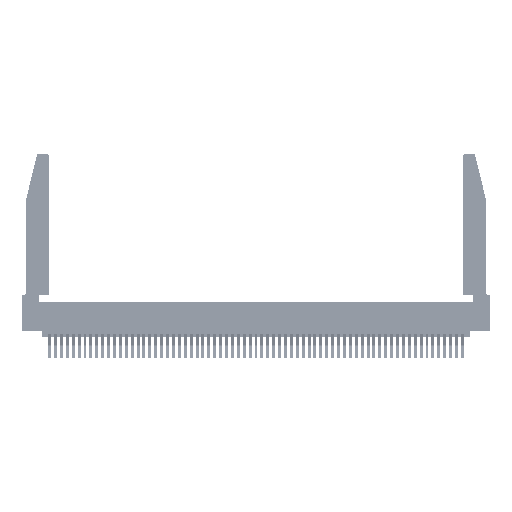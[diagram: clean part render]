
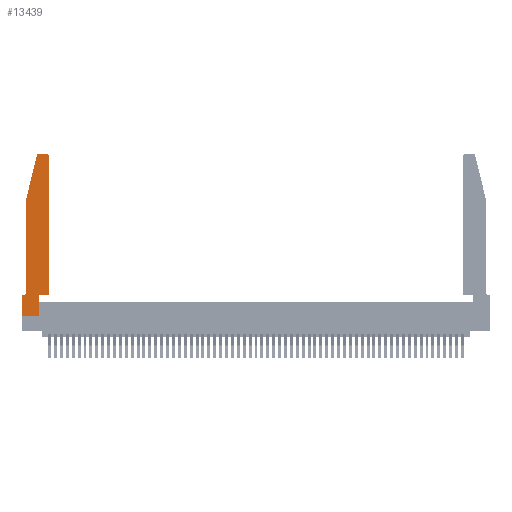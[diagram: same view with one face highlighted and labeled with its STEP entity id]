
A CAD part, top view. The second image highlights one B-rep face of the part: STEP entity #13439.
In plain terms, the highlighted planar face has unit normal (0, 0, 1).
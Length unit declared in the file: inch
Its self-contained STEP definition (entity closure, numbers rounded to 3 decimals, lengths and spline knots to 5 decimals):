
#87 = ORIENTED_EDGE ( 'NONE', *, *, #21274, .T. ) ;
#419 = VECTOR ( 'NONE', #16377, 39.37008 ) ;
#1144 = VERTEX_POINT ( 'NONE', #14905 ) ;
#1834 = CARTESIAN_POINT ( 'NONE',  ( 0.0055, 0.35, 0.37 ) ) ;
#1866 = LINE ( 'NONE', #2980, #419 ) ;
#2343 = EDGE_CURVE ( 'NONE', #43967, #1144, #30442, .T. ) ;
#2518 = CARTESIAN_POINT ( 'NONE',  ( 0.2865, 0.35, 0.37 ) ) ;
#2842 = ORIENTED_EDGE ( 'NONE', *, *, #17449, .T. ) ;
#2980 = CARTESIAN_POINT ( 'NONE',  ( 0.4505, 0.35, 0.37 ) ) ;
#3191 = LINE ( 'NONE', #33916, #36952 ) ;
#3892 = CARTESIAN_POINT ( 'NONE',  ( 0., 0.35, 0.37 ) ) ;
#4435 = DIRECTION ( 'NONE',  ( 1., 0., 0. ) ) ;
#4723 = CARTESIAN_POINT ( 'NONE',  ( 0.0755, 0.35, 0.37 ) ) ;
#4986 = EDGE_CURVE ( 'NONE', #23277, #34594, #48489, .T. ) ;
#5248 = CIRCLE ( 'NONE', #18675, 0.03 ) ;
#5651 = CARTESIAN_POINT ( 'NONE',  ( 0., 0., 0.37 ) ) ;
#5945 = CARTESIAN_POINT ( 'NONE',  ( 0.4205, 2.75, 0.37 ) ) ;
#7205 = ORIENTED_EDGE ( 'NONE', *, *, #27578, .T. ) ;
#7574 = DIRECTION ( 'NONE',  ( 0., -1., 0. ) ) ;
#7588 = PLANE ( 'NONE',  #23251 ) ;
#9173 = DIRECTION ( 'NONE',  ( -1., 0., 0. ) ) ;
#9368 = CARTESIAN_POINT ( 'NONE',  ( 0.284, 2.72, 0.37 ) ) ;
#11426 = CARTESIAN_POINT ( 'NONE',  ( 0.4505, 2.72, 0.37 ) ) ;
#11681 = ORIENTED_EDGE ( 'NONE', *, *, #2343, .T. ) ;
#11766 = ORIENTED_EDGE ( 'NONE', *, *, #26787, .T. ) ;
#12074 = CARTESIAN_POINT ( 'NONE',  ( 0., 0.35, 0.37 ) ) ;
#12823 = CIRCLE ( 'NONE', #55112, 0.03 ) ;
#13439 = ADVANCED_FACE ( 'NONE', ( #52415 ), #7588, .T. ) ;
#13842 = DIRECTION ( 'NONE',  ( 1., 0., 0. ) ) ;
#14390 = DIRECTION ( 'NONE',  ( -0.239, -0.971, 0. ) ) ;
#14905 = CARTESIAN_POINT ( 'NONE',  ( 0.0755, 2., 0.37 ) ) ;
#14991 = VECTOR ( 'NONE', #24948, 39.37008 ) ;
#16377 = DIRECTION ( 'NONE',  ( 0., 1., 0. ) ) ;
#16488 = CARTESIAN_POINT ( 'NONE',  ( 0.0755, 0.42, 0.37 ) ) ;
#16492 = DIRECTION ( 'NONE',  ( 1., 0., 0. ) ) ;
#17449 = EDGE_CURVE ( 'NONE', #37612, #43967, #12823, .T. ) ;
#18675 = AXIS2_PLACEMENT_3D ( 'NONE', #40758, #30841, #4435 ) ;
#18746 = VECTOR ( 'NONE', #14390, 39.37008 ) ;
#18855 = VERTEX_POINT ( 'NONE', #45283 ) ;
#19346 = VECTOR ( 'NONE', #50875, 39.37008 ) ;
#19733 = CARTESIAN_POINT ( 'NONE',  ( 0.284, 2.75, 0.37 ) ) ;
#19841 = VERTEX_POINT ( 'NONE', #5945 ) ;
#19895 = DIRECTION ( 'NONE',  ( 1., 0., 0. ) ) ;
#21274 = EDGE_CURVE ( 'NONE', #1144, #23277, #3191, .T. ) ;
#21321 = DIRECTION ( 'NONE',  ( 1., 0., 0. ) ) ;
#21453 = EDGE_CURVE ( 'NONE', #52784, #19841, #5248, .T. ) ;
#21777 = CARTESIAN_POINT ( 'NONE',  ( 0.25487, 2.72718, 0.37 ) ) ;
#21817 = EDGE_CURVE ( 'NONE', #27406, #36793, #34089, .T. ) ;
#22331 = ORIENTED_EDGE ( 'NONE', *, *, #37382, .T. ) ;
#22633 = ORIENTED_EDGE ( 'NONE', *, *, #4986, .T. ) ;
#23251 = AXIS2_PLACEMENT_3D ( 'NONE', #12074, #42696, #16492 ) ;
#23277 = VERTEX_POINT ( 'NONE', #16488 ) ;
#24948 = DIRECTION ( 'NONE',  ( -1., 0., 0. ) ) ;
#25304 = LINE ( 'NONE', #51031, #14991 ) ;
#25849 = ORIENTED_EDGE ( 'NONE', *, *, #21817, .T. ) ;
#26250 = CARTESIAN_POINT ( 'NONE',  ( 0.0055, 0.42, 0.37 ) ) ;
#26787 = EDGE_CURVE ( 'NONE', #36793, #52784, #1866, .T. ) ;
#27406 = VERTEX_POINT ( 'NONE', #2518 ) ;
#27530 = ORIENTED_EDGE ( 'NONE', *, *, #21453, .T. ) ;
#27578 = EDGE_CURVE ( 'NONE', #53768, #18855, #29294, .T. ) ;
#28714 = CARTESIAN_POINT ( 'NONE',  ( 0.4505, 0.35, 0.37 ) ) ;
#29047 = LINE ( 'NONE', #4723, #39296 ) ;
#29294 = LINE ( 'NONE', #55948, #42261 ) ;
#29389 = CARTESIAN_POINT ( 'NONE',  ( 0.2865, 0.35, 0.37 ) ) ;
#30442 = LINE ( 'NONE', #36247, #18746 ) ;
#30656 = DIRECTION ( 'NONE',  ( -1., 0., 0. ) ) ;
#30841 = DIRECTION ( 'NONE',  ( 0., 0., 1. ) ) ;
#32003 = ORIENTED_EDGE ( 'NONE', *, *, #48124, .T. ) ;
#32710 = ORIENTED_EDGE ( 'NONE', *, *, #39505, .T. ) ;
#33187 = LINE ( 'NONE', #54796, #53584 ) ;
#33916 = CARTESIAN_POINT ( 'NONE',  ( 0.0755, 2., 0.37 ) ) ;
#34089 = LINE ( 'NONE', #28714, #45674 ) ;
#34560 = CARTESIAN_POINT ( 'NONE',  ( 0.4505, 0.35, 0.37 ) ) ;
#34594 = VERTEX_POINT ( 'NONE', #1834 ) ;
#34675 = ORIENTED_EDGE ( 'NONE', *, *, #51251, .T. ) ;
#36247 = CARTESIAN_POINT ( 'NONE',  ( 0.0755, 2., 0.37 ) ) ;
#36793 = VERTEX_POINT ( 'NONE', #34560 ) ;
#36952 = VECTOR ( 'NONE', #7574, 39.37008 ) ;
#37382 = EDGE_CURVE ( 'NONE', #18855, #27406, #41230, .T. ) ;
#37612 = VERTEX_POINT ( 'NONE', #19733 ) ;
#39296 = VECTOR ( 'NONE', #9173, 39.37008 ) ;
#39505 = EDGE_CURVE ( 'NONE', #44656, #53768, #33187, .T. ) ;
#40082 = DIRECTION ( 'NONE',  ( 0., 0., 1. ) ) ;
#40758 = CARTESIAN_POINT ( 'NONE',  ( 0.4205, 2.72, 0.37 ) ) ;
#41230 = LINE ( 'NONE', #29389, #19346 ) ;
#42261 = VECTOR ( 'NONE', #21321, 39.37008 ) ;
#42476 = EDGE_LOOP ( 'NONE', ( #32003, #2842, #11681, #87, #22633, #34675, #32710, #7205, #22331, #25849, #11766, #27530 ) ) ;
#42696 = DIRECTION ( 'NONE',  ( 0., 0., 1. ) ) ;
#43967 = VERTEX_POINT ( 'NONE', #21777 ) ;
#44656 = VERTEX_POINT ( 'NONE', #3892 ) ;
#45283 = CARTESIAN_POINT ( 'NONE',  ( 0.2865, 0., 0.37 ) ) ;
#45674 = VECTOR ( 'NONE', #19895, 39.37008 ) ;
#46716 = AXIS2_PLACEMENT_3D ( 'NONE', #26250, #56652, #30656 ) ;
#48124 = EDGE_CURVE ( 'NONE', #19841, #37612, #25304, .T. ) ;
#48489 = CIRCLE ( 'NONE', #46716, 0.07 ) ;
#50613 = DIRECTION ( 'NONE',  ( 0., -1., 0. ) ) ;
#50875 = DIRECTION ( 'NONE',  ( 0., 1., 0. ) ) ;
#51031 = CARTESIAN_POINT ( 'NONE',  ( 0.2605, 2.75, 0.37 ) ) ;
#51251 = EDGE_CURVE ( 'NONE', #34594, #44656, #29047, .T. ) ;
#52415 = FACE_OUTER_BOUND ( 'NONE', #42476, .T. ) ;
#52784 = VERTEX_POINT ( 'NONE', #11426 ) ;
#53584 = VECTOR ( 'NONE', #50613, 39.37008 ) ;
#53768 = VERTEX_POINT ( 'NONE', #5651 ) ;
#54796 = CARTESIAN_POINT ( 'NONE',  ( 0., 0., 0.37 ) ) ;
#55112 = AXIS2_PLACEMENT_3D ( 'NONE', #9368, #40082, #13842 ) ;
#55948 = CARTESIAN_POINT ( 'NONE',  ( 0., 0., 0.37 ) ) ;
#56652 = DIRECTION ( 'NONE',  ( 0., 0., -1. ) ) ;
